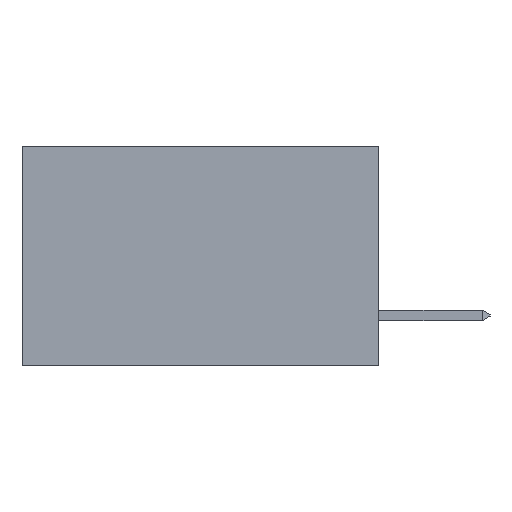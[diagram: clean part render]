
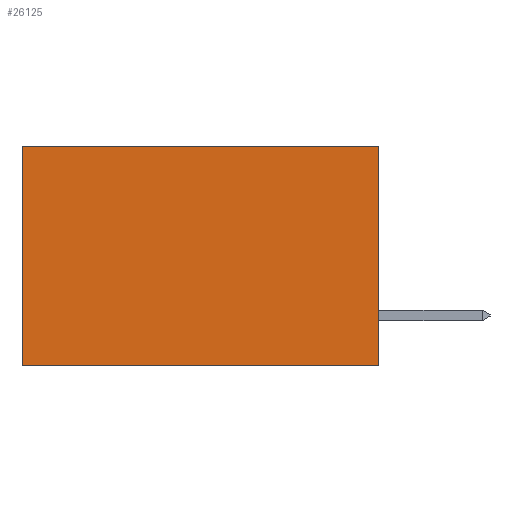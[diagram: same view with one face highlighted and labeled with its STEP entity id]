
A CAD part, left-side view. The second image highlights one B-rep face of the part: STEP entity #26125.
In plain terms, the highlighted planar face has unit normal (-1, 0, 0).
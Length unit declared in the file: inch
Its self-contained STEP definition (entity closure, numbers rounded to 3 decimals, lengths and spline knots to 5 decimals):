
#47 = VECTOR ( 'NONE', #26972, 39.37008 ) ;
#3771 = CARTESIAN_POINT ( 'NONE',  ( 0.298, 0., -0.37 ) ) ;
#3963 = PLANE ( 'NONE',  #7227 ) ;
#5743 = LINE ( 'NONE', #25833, #15849 ) ;
#5837 = CARTESIAN_POINT ( 'NONE',  ( 0.298, 0., 0. ) ) ;
#6089 = FACE_OUTER_BOUND ( 'NONE', #18415, .T. ) ;
#6106 = DIRECTION ( 'NONE',  ( 0., 0., -1. ) ) ;
#6338 = LINE ( 'NONE', #3771, #47 ) ;
#6743 = CARTESIAN_POINT ( 'NONE',  ( 0.298, 0.6, -0.37 ) ) ;
#7227 = AXIS2_PLACEMENT_3D ( 'NONE', #25119, #18929, #6106 ) ;
#7476 = CARTESIAN_POINT ( 'NONE',  ( 0.298, 0.6, 0. ) ) ;
#10298 = ORIENTED_EDGE ( 'NONE', *, *, #15029, .F. ) ;
#10387 = EDGE_CURVE ( 'NONE', #22778, #12741, #6338, .T. ) ;
#11483 = CARTESIAN_POINT ( 'NONE',  ( 0.298, 0., 0. ) ) ;
#12666 = CARTESIAN_POINT ( 'NONE',  ( 0.298, 0., -0.37 ) ) ;
#12736 = CARTESIAN_POINT ( 'NONE',  ( 0.298, 0., 0. ) ) ;
#12741 = VERTEX_POINT ( 'NONE', #6743 ) ;
#12971 = VERTEX_POINT ( 'NONE', #7476 ) ;
#14189 = ORIENTED_EDGE ( 'NONE', *, *, #10387, .F. ) ;
#15029 = EDGE_CURVE ( 'NONE', #19912, #22778, #25769, .T. ) ;
#15849 = VECTOR ( 'NONE', #17566, 39.37008 ) ;
#16196 = ORIENTED_EDGE ( 'NONE', *, *, #25568, .T. ) ;
#16551 = VECTOR ( 'NONE', #16890, 39.37008 ) ;
#16890 = DIRECTION ( 'NONE',  ( 0., 1., 0. ) ) ;
#17566 = DIRECTION ( 'NONE',  ( 0., 0., -1. ) ) ;
#18415 = EDGE_LOOP ( 'NONE', ( #20306, #14189, #10298, #16196 ) ) ;
#18929 = DIRECTION ( 'NONE',  ( 1., 0., 0. ) ) ;
#19912 = VERTEX_POINT ( 'NONE', #11483 ) ;
#20241 = VECTOR ( 'NONE', #26993, 39.37008 ) ;
#20306 = ORIENTED_EDGE ( 'NONE', *, *, #26332, .T. ) ;
#22778 = VERTEX_POINT ( 'NONE', #12666 ) ;
#25119 = CARTESIAN_POINT ( 'NONE',  ( 0.298, 0., 0. ) ) ;
#25568 = EDGE_CURVE ( 'NONE', #19912, #12971, #26946, .T. ) ;
#25769 = LINE ( 'NONE', #5837, #20241 ) ;
#25833 = CARTESIAN_POINT ( 'NONE',  ( 0.298, 0.6, 0. ) ) ;
#26125 = ADVANCED_FACE ( 'NONE', ( #6089 ), #3963, .F. ) ;
#26332 = EDGE_CURVE ( 'NONE', #12971, #12741, #5743, .T. ) ;
#26946 = LINE ( 'NONE', #12736, #16551 ) ;
#26972 = DIRECTION ( 'NONE',  ( 0., 1., 0. ) ) ;
#26993 = DIRECTION ( 'NONE',  ( 0., 0., -1. ) ) ;
